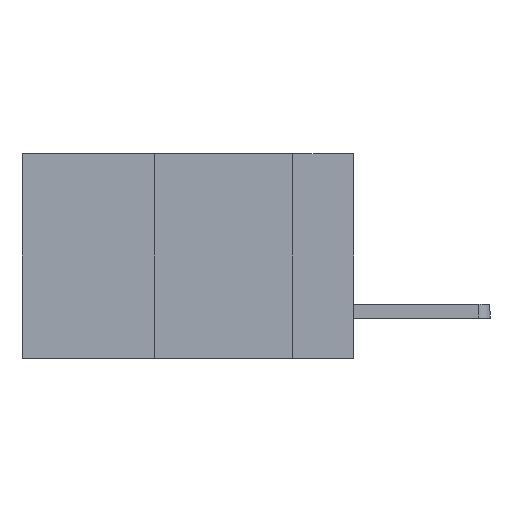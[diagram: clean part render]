
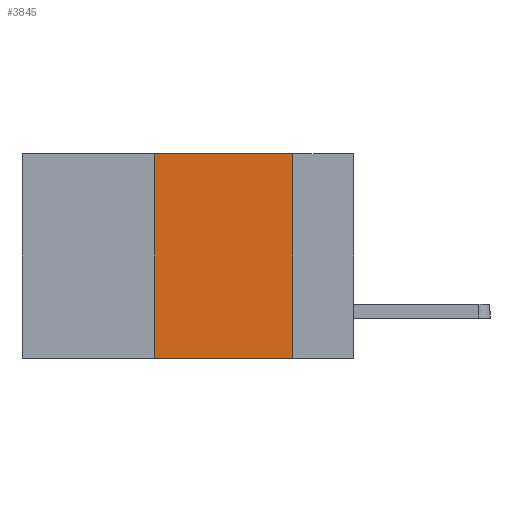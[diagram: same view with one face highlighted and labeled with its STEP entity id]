
A CAD part, left-side view. The second image highlights one B-rep face of the part: STEP entity #3845.
In plain terms, the highlighted planar face has unit normal (-1, 0, 0).
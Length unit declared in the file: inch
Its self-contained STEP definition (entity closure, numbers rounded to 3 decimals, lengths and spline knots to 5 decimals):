
#352 = DIRECTION ( 'NONE',  ( 0., 0., -1. ) ) ;
#433 = CARTESIAN_POINT ( 'NONE',  ( 0., 0.11, 0. ) ) ;
#829 = EDGE_CURVE ( 'NONE', #9584, #7205, #4034, .T. ) ;
#887 = EDGE_LOOP ( 'NONE', ( #1503, #5935, #8257, #5029 ) ) ;
#1503 = ORIENTED_EDGE ( 'NONE', *, *, #4207, .F. ) ;
#1608 = VECTOR ( 'NONE', #8980, 39.37008 ) ;
#1830 = FACE_OUTER_BOUND ( 'NONE', #887, .T. ) ;
#2171 = VECTOR ( 'NONE', #7321, 39.37008 ) ;
#2361 = VERTEX_POINT ( 'NONE', #9270 ) ;
#2370 = EDGE_CURVE ( 'NONE', #2361, #2621, #4225, .T. ) ;
#2380 = EDGE_CURVE ( 'NONE', #2361, #9584, #3717, .T. ) ;
#2621 = VERTEX_POINT ( 'NONE', #7269 ) ;
#2745 = AXIS2_PLACEMENT_3D ( 'NONE', #3735, #3558, #3549 ) ;
#2792 = LINE ( 'NONE', #433, #6664 ) ;
#3359 = CARTESIAN_POINT ( 'NONE',  ( 0., 0.11, 0. ) ) ;
#3549 = DIRECTION ( 'NONE',  ( 0., 0., -1. ) ) ;
#3558 = DIRECTION ( 'NONE',  ( 1., 0., 0. ) ) ;
#3717 = LINE ( 'NONE', #9008, #1608 ) ;
#3735 = CARTESIAN_POINT ( 'NONE',  ( 0., 0.6, 0. ) ) ;
#3824 = PLANE ( 'NONE',  #2745 ) ;
#3845 = ADVANCED_FACE ( 'NONE', ( #1830 ), #3824, .F. ) ;
#4034 = LINE ( 'NONE', #7854, #2171 ) ;
#4207 = EDGE_CURVE ( 'NONE', #7205, #2621, #2792, .T. ) ;
#4225 = LINE ( 'NONE', #9101, #5799 ) ;
#5029 = ORIENTED_EDGE ( 'NONE', *, *, #2370, .T. ) ;
#5799 = VECTOR ( 'NONE', #9448, 39.37008 ) ;
#5935 = ORIENTED_EDGE ( 'NONE', *, *, #829, .F. ) ;
#6033 = CARTESIAN_POINT ( 'NONE',  ( 0., 0.36, 0. ) ) ;
#6664 = VECTOR ( 'NONE', #352, 39.37008 ) ;
#7205 = VERTEX_POINT ( 'NONE', #3359 ) ;
#7269 = CARTESIAN_POINT ( 'NONE',  ( 0., 0.11, -0.37 ) ) ;
#7321 = DIRECTION ( 'NONE',  ( 0., -1., 0. ) ) ;
#7854 = CARTESIAN_POINT ( 'NONE',  ( 0., 0.6, 0. ) ) ;
#8257 = ORIENTED_EDGE ( 'NONE', *, *, #2380, .F. ) ;
#8980 = DIRECTION ( 'NONE',  ( 0., 0., 1. ) ) ;
#9008 = CARTESIAN_POINT ( 'NONE',  ( 0., 0.36, 0. ) ) ;
#9101 = CARTESIAN_POINT ( 'NONE',  ( 0., 0.6, -0.37 ) ) ;
#9270 = CARTESIAN_POINT ( 'NONE',  ( 0., 0.36, -0.37 ) ) ;
#9448 = DIRECTION ( 'NONE',  ( 0., -1., 0. ) ) ;
#9584 = VERTEX_POINT ( 'NONE', #6033 ) ;
